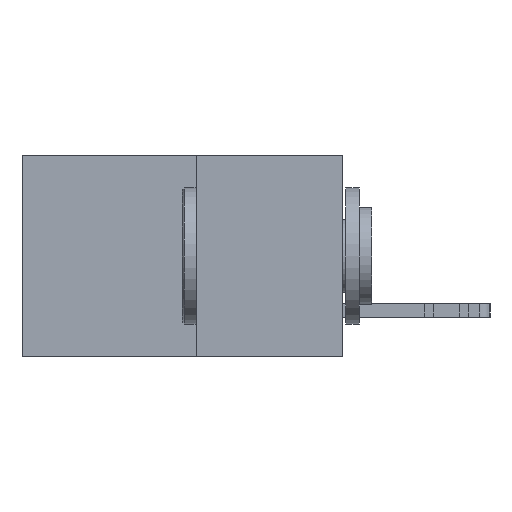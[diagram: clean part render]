
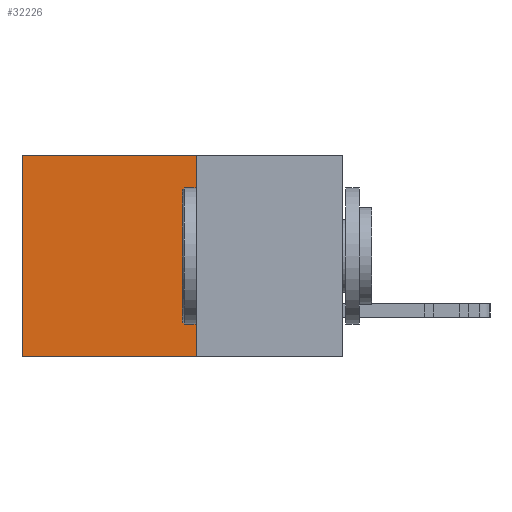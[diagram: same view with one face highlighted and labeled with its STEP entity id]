
A CAD part, left-side view. The second image highlights one B-rep face of the part: STEP entity #32226.
In plain terms, the highlighted planar face has unit normal (-1, 0, 0).
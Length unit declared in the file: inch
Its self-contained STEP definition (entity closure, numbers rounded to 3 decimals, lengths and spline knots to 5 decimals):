
#126 = CARTESIAN_POINT ( 'NONE',  ( 0.277, 0.27, -0.37 ) ) ;
#254 = ORIENTED_EDGE ( 'NONE', *, *, #28347, .T. ) ;
#859 = DIRECTION ( 'NONE',  ( 0., 0., -1. ) ) ;
#1474 = EDGE_CURVE ( 'NONE', #6012, #5961, #32894, .T. ) ;
#2754 = ORIENTED_EDGE ( 'NONE', *, *, #30194, .F. ) ;
#3324 = EDGE_LOOP ( 'NONE', ( #254, #25568, #2754, #27836 ) ) ;
#4399 = VERTEX_POINT ( 'NONE', #26667 ) ;
#4800 = PLANE ( 'NONE',  #15161 ) ;
#5698 = VERTEX_POINT ( 'NONE', #126 ) ;
#5961 = VERTEX_POINT ( 'NONE', #6341 ) ;
#6012 = VERTEX_POINT ( 'NONE', #19413 ) ;
#6341 = CARTESIAN_POINT ( 'NONE',  ( 0.277, 0.59, 0. ) ) ;
#6751 = VECTOR ( 'NONE', #25273, 39.37008 ) ;
#7300 = CARTESIAN_POINT ( 'NONE',  ( 0.277, 0.27, -0.37 ) ) ;
#7394 = DIRECTION ( 'NONE',  ( 1., 0., 0. ) ) ;
#7810 = DIRECTION ( 'NONE',  ( 0., 1., 0. ) ) ;
#10410 = CARTESIAN_POINT ( 'NONE',  ( 0.277, 0.27, -0.37 ) ) ;
#12394 = CARTESIAN_POINT ( 'NONE',  ( 0.277, 0.27, -0.37 ) ) ;
#15161 = AXIS2_PLACEMENT_3D ( 'NONE', #12394, #7394, #25378 ) ;
#18621 = LINE ( 'NONE', #31714, #24587 ) ;
#19244 = VECTOR ( 'NONE', #29615, 39.37008 ) ;
#19413 = CARTESIAN_POINT ( 'NONE',  ( 0.277, 0.27, 0. ) ) ;
#19469 = VECTOR ( 'NONE', #7810, 39.37008 ) ;
#20261 = LINE ( 'NONE', #10410, #19469 ) ;
#24587 = VECTOR ( 'NONE', #859, 39.37008 ) ;
#25273 = DIRECTION ( 'NONE',  ( 0., 0., -1. ) ) ;
#25378 = DIRECTION ( 'NONE',  ( 0., 0., -1. ) ) ;
#25568 = ORIENTED_EDGE ( 'NONE', *, *, #27395, .F. ) ;
#26667 = CARTESIAN_POINT ( 'NONE',  ( 0.277, 0.59, -0.37 ) ) ;
#27395 = EDGE_CURVE ( 'NONE', #5698, #4399, #20261, .T. ) ;
#27836 = ORIENTED_EDGE ( 'NONE', *, *, #1474, .T. ) ;
#28347 = EDGE_CURVE ( 'NONE', #5961, #4399, #18621, .T. ) ;
#29615 = DIRECTION ( 'NONE',  ( 0., 1., 0. ) ) ;
#29658 = CARTESIAN_POINT ( 'NONE',  ( 0.277, 0.27, 0. ) ) ;
#30194 = EDGE_CURVE ( 'NONE', #6012, #5698, #33318, .T. ) ;
#30372 = FACE_OUTER_BOUND ( 'NONE', #3324, .T. ) ;
#31714 = CARTESIAN_POINT ( 'NONE',  ( 0.277, 0.59, -0.37 ) ) ;
#32226 = ADVANCED_FACE ( 'NONE', ( #30372 ), #4800, .F. ) ;
#32894 = LINE ( 'NONE', #29658, #19244 ) ;
#33318 = LINE ( 'NONE', #7300, #6751 ) ;
